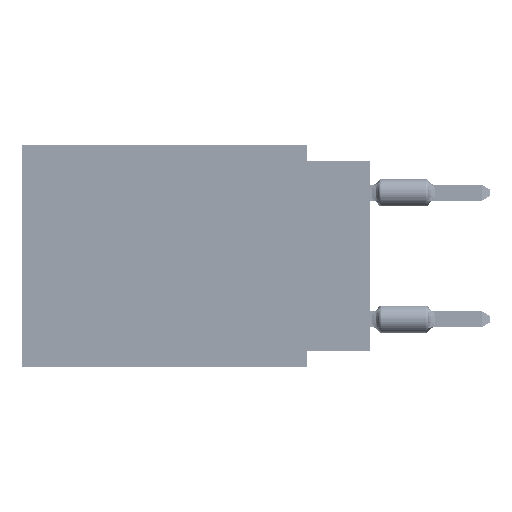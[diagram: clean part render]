
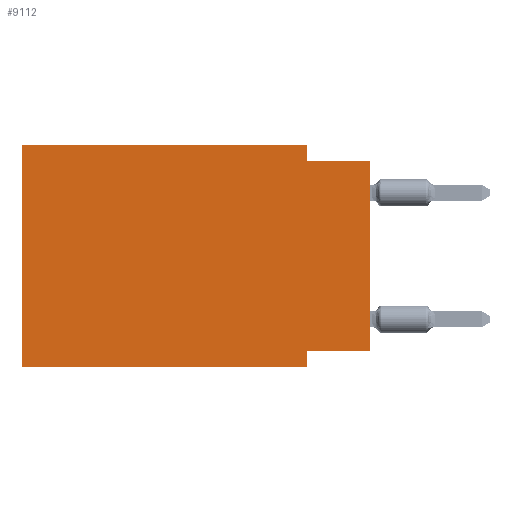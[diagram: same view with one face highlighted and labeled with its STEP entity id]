
A CAD part, left-side view. The second image highlights one B-rep face of the part: STEP entity #9112.
In plain terms, the highlighted planar face has unit normal (-1, 0, 0).
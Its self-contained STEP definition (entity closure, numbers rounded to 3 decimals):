
#225 = DIRECTION ( 'NONE',  ( 0., -1., 0. ) ) ;
#1406 = EDGE_CURVE ( 'NONE', #10603, #44705, #34883, .T. ) ;
#1874 = VECTOR ( 'NONE', #55788, 1000. ) ;
#2701 = VERTEX_POINT ( 'NONE', #9479 ) ;
#3253 = CARTESIAN_POINT ( 'NONE',  ( 0., 2.54, 0. ) ) ;
#3495 = ORIENTED_EDGE ( 'NONE', *, *, #8361, .F. ) ;
#3600 = LINE ( 'NONE', #3253, #6911 ) ;
#4573 = EDGE_CURVE ( 'NONE', #68401, #14184, #28008, .T. ) ;
#4800 = CARTESIAN_POINT ( 'NONE',  ( 0., 2.54, 0. ) ) ;
#4996 = CARTESIAN_POINT ( 'NONE',  ( 0., 2.54, -8.89 ) ) ;
#6296 = DIRECTION ( 'NONE',  ( 1., 0., 0. ) ) ;
#6911 = VECTOR ( 'NONE', #19337, 1000. ) ;
#8181 = ORIENTED_EDGE ( 'NONE', *, *, #4573, .F. ) ;
#8361 = EDGE_CURVE ( 'NONE', #44705, #68401, #3600, .T. ) ;
#9112 = ADVANCED_FACE ( 'NONE', ( #18352 ), #24190, .F. ) ;
#9479 = CARTESIAN_POINT ( 'NONE',  ( 0., 2.54, -8.255 ) ) ;
#9743 = CARTESIAN_POINT ( 'NONE',  ( 0., 2.54, -0.635 ) ) ;
#9823 = VECTOR ( 'NONE', #50423, 1000. ) ;
#9863 = ORIENTED_EDGE ( 'NONE', *, *, #16554, .F. ) ;
#10603 = VERTEX_POINT ( 'NONE', #52909 ) ;
#13151 = LINE ( 'NONE', #28891, #9823 ) ;
#13191 = VECTOR ( 'NONE', #22160, 1000. ) ;
#13341 = ORIENTED_EDGE ( 'NONE', *, *, #21675, .F. ) ;
#14184 = VERTEX_POINT ( 'NONE', #60284 ) ;
#16554 = EDGE_CURVE ( 'NONE', #43377, #2701, #47590, .T. ) ;
#16687 = ORIENTED_EDGE ( 'NONE', *, *, #53983, .T. ) ;
#18352 = FACE_OUTER_BOUND ( 'NONE', #25070, .T. ) ;
#19337 = DIRECTION ( 'NONE',  ( 0., 0., -1. ) ) ;
#21675 = EDGE_CURVE ( 'NONE', #2701, #58146, #21818, .T. ) ;
#21818 = LINE ( 'NONE', #4996, #13191 ) ;
#22160 = DIRECTION ( 'NONE',  ( 0., 0., -1. ) ) ;
#23455 = CARTESIAN_POINT ( 'NONE',  ( 0., 13.97, 0. ) ) ;
#24190 = PLANE ( 'NONE',  #55979 ) ;
#25070 = EDGE_LOOP ( 'NONE', ( #39913, #8181, #3495, #26681, #26548, #16687, #13341, #9863 ) ) ;
#26548 = ORIENTED_EDGE ( 'NONE', *, *, #48442, .F. ) ;
#26681 = ORIENTED_EDGE ( 'NONE', *, *, #1406, .F. ) ;
#27062 = CARTESIAN_POINT ( 'NONE',  ( 0., 0., -8.255 ) ) ;
#27873 = CARTESIAN_POINT ( 'NONE',  ( 0., 13.97, -8.89 ) ) ;
#28008 = LINE ( 'NONE', #38229, #43896 ) ;
#28716 = LINE ( 'NONE', #63037, #41134 ) ;
#28891 = CARTESIAN_POINT ( 'NONE',  ( 0., 0., 0. ) ) ;
#29410 = DIRECTION ( 'NONE',  ( 0., -1., 0. ) ) ;
#32770 = VECTOR ( 'NONE', #40651, 1000. ) ;
#34883 = LINE ( 'NONE', #68516, #51092 ) ;
#36635 = VERTEX_POINT ( 'NONE', #27873 ) ;
#38229 = CARTESIAN_POINT ( 'NONE',  ( 0., 0., -0.635 ) ) ;
#39913 = ORIENTED_EDGE ( 'NONE', *, *, #40368, .T. ) ;
#40368 = EDGE_CURVE ( 'NONE', #43377, #14184, #13151, .T. ) ;
#40651 = DIRECTION ( 'NONE',  ( 0., 1., 0. ) ) ;
#41134 = VECTOR ( 'NONE', #45140, 1000. ) ;
#43377 = VERTEX_POINT ( 'NONE', #27062 ) ;
#43896 = VECTOR ( 'NONE', #225, 1000. ) ;
#44705 = VERTEX_POINT ( 'NONE', #4800 ) ;
#45140 = DIRECTION ( 'NONE',  ( 0., 0., 1. ) ) ;
#47590 = LINE ( 'NONE', #62614, #32770 ) ;
#48442 = EDGE_CURVE ( 'NONE', #36635, #10603, #28716, .T. ) ;
#50423 = DIRECTION ( 'NONE',  ( 0., 0., 1. ) ) ;
#51092 = VECTOR ( 'NONE', #29410, 1000. ) ;
#52909 = CARTESIAN_POINT ( 'NONE',  ( 0., 13.97, 0. ) ) ;
#53983 = EDGE_CURVE ( 'NONE', #36635, #58146, #62366, .T. ) ;
#55788 = DIRECTION ( 'NONE',  ( 0., -1., 0. ) ) ;
#55979 = AXIS2_PLACEMENT_3D ( 'NONE', #23455, #6296, #62580 ) ;
#58146 = VERTEX_POINT ( 'NONE', #62760 ) ;
#60284 = CARTESIAN_POINT ( 'NONE',  ( 0., 0., -0.635 ) ) ;
#62366 = LINE ( 'NONE', #68195, #1874 ) ;
#62580 = DIRECTION ( 'NONE',  ( 0., 0., -1. ) ) ;
#62614 = CARTESIAN_POINT ( 'NONE',  ( 0., 0., -8.255 ) ) ;
#62760 = CARTESIAN_POINT ( 'NONE',  ( 0., 2.54, -8.89 ) ) ;
#63037 = CARTESIAN_POINT ( 'NONE',  ( 0., 13.97, 0. ) ) ;
#68195 = CARTESIAN_POINT ( 'NONE',  ( 0., 13.97, -8.89 ) ) ;
#68401 = VERTEX_POINT ( 'NONE', #9743 ) ;
#68516 = CARTESIAN_POINT ( 'NONE',  ( 0., 13.97, 0. ) ) ;
